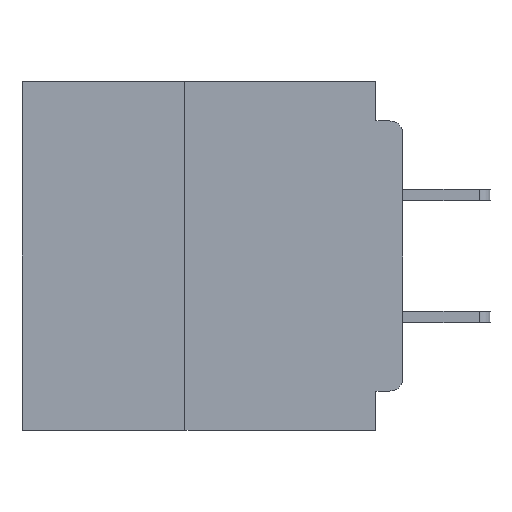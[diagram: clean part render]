
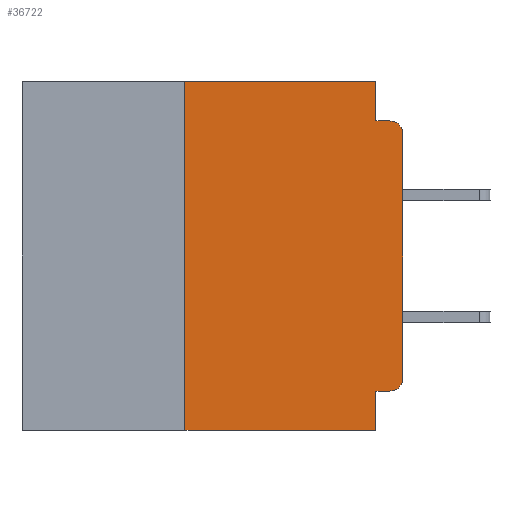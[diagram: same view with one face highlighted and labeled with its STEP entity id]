
A CAD part, left-side view. The second image highlights one B-rep face of the part: STEP entity #36722.
In plain terms, the highlighted planar face has unit normal (-1, 0, 0).
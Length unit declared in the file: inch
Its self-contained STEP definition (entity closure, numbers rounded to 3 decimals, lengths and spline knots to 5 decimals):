
#634 = DIRECTION ( 'NONE',  ( -1., 0., 0. ) ) ;
#669 = CARTESIAN_POINT ( 'NONE',  ( 0., 0.25, -0.4 ) ) ;
#2253 = DIRECTION ( 'NONE',  ( 0., 0., -1. ) ) ;
#2404 = VECTOR ( 'NONE', #9843, 39.37008 ) ;
#4409 = DIRECTION ( 'NONE',  ( 0., 0., 1. ) ) ;
#4749 = LINE ( 'NONE', #14688, #52975 ) ;
#5239 = VERTEX_POINT ( 'NONE', #46332 ) ;
#5396 = LINE ( 'NONE', #41135, #30332 ) ;
#5857 = DIRECTION ( 'NONE',  ( 0., 1., 0. ) ) ;
#6028 = VERTEX_POINT ( 'NONE', #29545 ) ;
#6402 = CARTESIAN_POINT ( 'NONE',  ( 0., 0., 0. ) ) ;
#7326 = CARTESIAN_POINT ( 'NONE',  ( 0., 0.031, -0.4 ) ) ;
#7689 = VERTEX_POINT ( 'NONE', #17254 ) ;
#7849 = VECTOR ( 'NONE', #5857, 39.37008 ) ;
#7925 = CARTESIAN_POINT ( 'NONE',  ( 0., 0.437, 0. ) ) ;
#8900 = VECTOR ( 'NONE', #12018, 39.37008 ) ;
#9843 = DIRECTION ( 'NONE',  ( 0., -1., 0. ) ) ;
#10405 = ORIENTED_EDGE ( 'NONE', *, *, #19280, .F. ) ;
#11212 = ORIENTED_EDGE ( 'NONE', *, *, #34791, .F. ) ;
#12018 = DIRECTION ( 'NONE',  ( 0., 0., -1. ) ) ;
#12367 = CARTESIAN_POINT ( 'NONE',  ( 0., 0., -0.34 ) ) ;
#13225 = EDGE_CURVE ( 'NONE', #7689, #18361, #37511, .T. ) ;
#14688 = CARTESIAN_POINT ( 'NONE',  ( 0., 0., -0.045 ) ) ;
#15189 = VECTOR ( 'NONE', #4409, 39.37008 ) ;
#15441 = EDGE_CURVE ( 'NONE', #53732, #57101, #57756, .T. ) ;
#15703 = EDGE_CURVE ( 'NONE', #18361, #25937, #43076, .T. ) ;
#15851 = VERTEX_POINT ( 'NONE', #49516 ) ;
#17254 = CARTESIAN_POINT ( 'NONE',  ( 0., 0.015, -0.355 ) ) ;
#17326 = DIRECTION ( 'NONE',  ( 0., 0., -1. ) ) ;
#17850 = EDGE_LOOP ( 'NONE', ( #35208, #37186, #10405, #53873, #57395, #11212, #18635, #25762, #46248, #36136 ) ) ;
#18361 = VERTEX_POINT ( 'NONE', #12367 ) ;
#18635 = ORIENTED_EDGE ( 'NONE', *, *, #38116, .T. ) ;
#18777 = CARTESIAN_POINT ( 'NONE',  ( 0., 0.031, -0.045 ) ) ;
#19280 = EDGE_CURVE ( 'NONE', #57101, #15851, #4749, .T. ) ;
#19718 = AXIS2_PLACEMENT_3D ( 'NONE', #28684, #634, #33378 ) ;
#20276 = LINE ( 'NONE', #24493, #7849 ) ;
#20447 = VERTEX_POINT ( 'NONE', #669 ) ;
#21191 = VERTEX_POINT ( 'NONE', #28627 ) ;
#22060 = CARTESIAN_POINT ( 'NONE',  ( 0., 0.031, 0. ) ) ;
#24128 = DIRECTION ( 'NONE',  ( 0., -1., 0. ) ) ;
#24493 = CARTESIAN_POINT ( 'NONE',  ( 0., 0., -0.355 ) ) ;
#25762 = ORIENTED_EDGE ( 'NONE', *, *, #39060, .F. ) ;
#25937 = VERTEX_POINT ( 'NONE', #53734 ) ;
#27763 = CARTESIAN_POINT ( 'NONE',  ( 0., 0.25, -0.4 ) ) ;
#28627 = CARTESIAN_POINT ( 'NONE',  ( 0., 0.031, -0.355 ) ) ;
#28684 = CARTESIAN_POINT ( 'NONE',  ( 0., 0.015, -0.34 ) ) ;
#28721 = DIRECTION ( 'NONE',  ( 0., 0., 1. ) ) ;
#29545 = CARTESIAN_POINT ( 'NONE',  ( 0., 0.031, -0.4 ) ) ;
#30332 = VECTOR ( 'NONE', #50368, 39.37008 ) ;
#30347 = DIRECTION ( 'NONE',  ( -1., 0., 0. ) ) ;
#31531 = VECTOR ( 'NONE', #45865, 39.37008 ) ;
#31837 = CARTESIAN_POINT ( 'NONE',  ( 0., 0.031, 0. ) ) ;
#32355 = LINE ( 'NONE', #7326, #8900 ) ;
#33180 = CARTESIAN_POINT ( 'NONE',  ( 0., 0.437, -0.4 ) ) ;
#33378 = DIRECTION ( 'NONE',  ( 0., 0., -1. ) ) ;
#34791 = EDGE_CURVE ( 'NONE', #20447, #5239, #52458, .T. ) ;
#35208 = ORIENTED_EDGE ( 'NONE', *, *, #15703, .T. ) ;
#35359 = LINE ( 'NONE', #33180, #2404 ) ;
#36136 = ORIENTED_EDGE ( 'NONE', *, *, #13225, .T. ) ;
#36722 = ADVANCED_FACE ( 'NONE', ( #53777 ), #59172, .F. ) ;
#37186 = ORIENTED_EDGE ( 'NONE', *, *, #38366, .T. ) ;
#37390 = AXIS2_PLACEMENT_3D ( 'NONE', #7925, #45324, #17326 ) ;
#37511 = CIRCLE ( 'NONE', #19718, 0.015 ) ;
#38116 = EDGE_CURVE ( 'NONE', #20447, #6028, #35359, .T. ) ;
#38366 = EDGE_CURVE ( 'NONE', #25937, #15851, #47016, .T. ) ;
#39060 = EDGE_CURVE ( 'NONE', #21191, #6028, #32355, .T. ) ;
#40595 = AXIS2_PLACEMENT_3D ( 'NONE', #58242, #30347, #2253 ) ;
#41135 = CARTESIAN_POINT ( 'NONE',  ( 0., 0.437, 0. ) ) ;
#43076 = LINE ( 'NONE', #6402, #54092 ) ;
#45324 = DIRECTION ( 'NONE',  ( 1., 0., 0. ) ) ;
#45865 = DIRECTION ( 'NONE',  ( 0., 0., -1. ) ) ;
#46248 = ORIENTED_EDGE ( 'NONE', *, *, #51586, .F. ) ;
#46332 = CARTESIAN_POINT ( 'NONE',  ( 0., 0.25, 0. ) ) ;
#47016 = CIRCLE ( 'NONE', #40595, 0.015 ) ;
#49516 = CARTESIAN_POINT ( 'NONE',  ( 0., 0.015, -0.045 ) ) ;
#50368 = DIRECTION ( 'NONE',  ( 0., -1., 0. ) ) ;
#51586 = EDGE_CURVE ( 'NONE', #7689, #21191, #20276, .T. ) ;
#52458 = LINE ( 'NONE', #27763, #15189 ) ;
#52975 = VECTOR ( 'NONE', #24128, 39.37008 ) ;
#53732 = VERTEX_POINT ( 'NONE', #22060 ) ;
#53734 = CARTESIAN_POINT ( 'NONE',  ( 0., 0., -0.06 ) ) ;
#53777 = FACE_OUTER_BOUND ( 'NONE', #17850, .T. ) ;
#53873 = ORIENTED_EDGE ( 'NONE', *, *, #15441, .F. ) ;
#54092 = VECTOR ( 'NONE', #28721, 39.37008 ) ;
#54434 = EDGE_CURVE ( 'NONE', #5239, #53732, #5396, .T. ) ;
#57101 = VERTEX_POINT ( 'NONE', #18777 ) ;
#57395 = ORIENTED_EDGE ( 'NONE', *, *, #54434, .F. ) ;
#57756 = LINE ( 'NONE', #31837, #31531 ) ;
#58242 = CARTESIAN_POINT ( 'NONE',  ( 0., 0.015, -0.06 ) ) ;
#59172 = PLANE ( 'NONE',  #37390 ) ;
